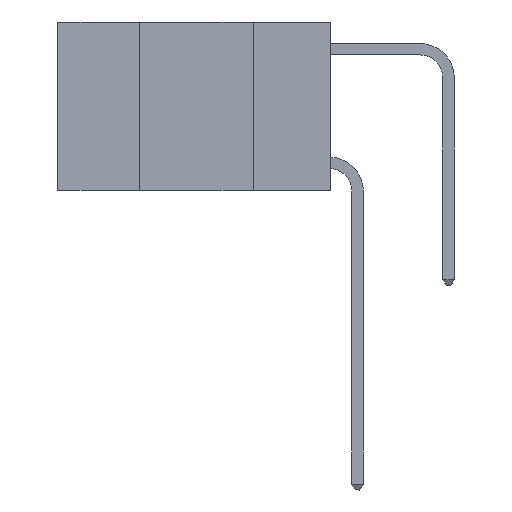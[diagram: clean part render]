
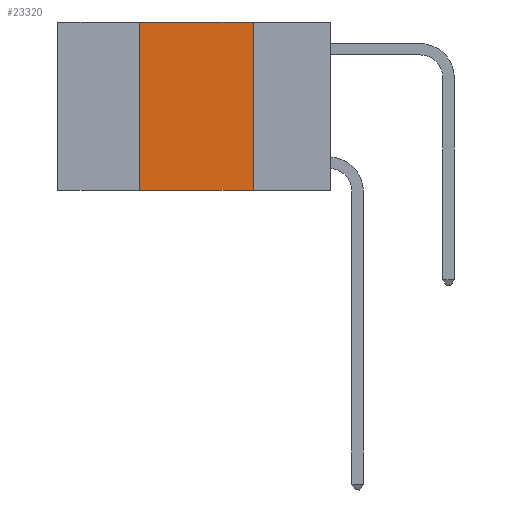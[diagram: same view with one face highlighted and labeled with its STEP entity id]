
A CAD part, left-side view. The second image highlights one B-rep face of the part: STEP entity #23320.
In plain terms, the highlighted planar face has unit normal (-1, 0, 0).
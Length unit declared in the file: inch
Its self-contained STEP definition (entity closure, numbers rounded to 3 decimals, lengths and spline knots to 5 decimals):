
#147 = EDGE_LOOP ( 'NONE', ( #21554, #1984, #15057, #363 ) ) ;
#363 = ORIENTED_EDGE ( 'NONE', *, *, #2647, .T. ) ;
#795 = VECTOR ( 'NONE', #6545, 39.37008 ) ;
#899 = LINE ( 'NONE', #19950, #795 ) ;
#912 = LINE ( 'NONE', #8408, #30719 ) ;
#1277 = PLANE ( 'NONE',  #8702 ) ;
#1789 = VERTEX_POINT ( 'NONE', #21101 ) ;
#1984 = ORIENTED_EDGE ( 'NONE', *, *, #3724, .F. ) ;
#2123 = CARTESIAN_POINT ( 'NONE',  ( 0., 0.6, -0.37 ) ) ;
#2647 = EDGE_CURVE ( 'NONE', #20685, #28170, #6988, .T. ) ;
#3724 = EDGE_CURVE ( 'NONE', #28452, #1789, #899, .T. ) ;
#5527 = DIRECTION ( 'NONE',  ( 0., 0., -1. ) ) ;
#6135 = CARTESIAN_POINT ( 'NONE',  ( 0., 0.6, 0. ) ) ;
#6545 = DIRECTION ( 'NONE',  ( 0., -1., 0. ) ) ;
#6682 = DIRECTION ( 'NONE',  ( 0., -1., 0. ) ) ;
#6988 = LINE ( 'NONE', #2123, #12580 ) ;
#8408 = CARTESIAN_POINT ( 'NONE',  ( 0., 0.17, 0. ) ) ;
#8702 = AXIS2_PLACEMENT_3D ( 'NONE', #6135, #22801, #5527 ) ;
#9055 = DIRECTION ( 'NONE',  ( 0., 0., 1. ) ) ;
#10368 = VECTOR ( 'NONE', #9055, 39.37008 ) ;
#12498 = EDGE_CURVE ( 'NONE', #20685, #28452, #30282, .T. ) ;
#12580 = VECTOR ( 'NONE', #6682, 39.37008 ) ;
#12905 = CARTESIAN_POINT ( 'NONE',  ( 0., 0.42, -0.37 ) ) ;
#15057 = ORIENTED_EDGE ( 'NONE', *, *, #12498, .F. ) ;
#16986 = CARTESIAN_POINT ( 'NONE',  ( 0., 0.17, -0.37 ) ) ;
#18425 = CARTESIAN_POINT ( 'NONE',  ( 0., 0.42, 0. ) ) ;
#19950 = CARTESIAN_POINT ( 'NONE',  ( 0., 0.6, 0. ) ) ;
#20009 = FACE_OUTER_BOUND ( 'NONE', #147, .T. ) ;
#20685 = VERTEX_POINT ( 'NONE', #12905 ) ;
#21101 = CARTESIAN_POINT ( 'NONE',  ( 0., 0.17, 0. ) ) ;
#21554 = ORIENTED_EDGE ( 'NONE', *, *, #29713, .F. ) ;
#22752 = DIRECTION ( 'NONE',  ( 0., 0., -1. ) ) ;
#22801 = DIRECTION ( 'NONE',  ( 1., 0., 0. ) ) ;
#22903 = CARTESIAN_POINT ( 'NONE',  ( 0., 0.42, 0. ) ) ;
#23320 = ADVANCED_FACE ( 'NONE', ( #20009 ), #1277, .F. ) ;
#28170 = VERTEX_POINT ( 'NONE', #16986 ) ;
#28452 = VERTEX_POINT ( 'NONE', #22903 ) ;
#29713 = EDGE_CURVE ( 'NONE', #1789, #28170, #912, .T. ) ;
#30282 = LINE ( 'NONE', #18425, #10368 ) ;
#30719 = VECTOR ( 'NONE', #22752, 39.37008 ) ;
